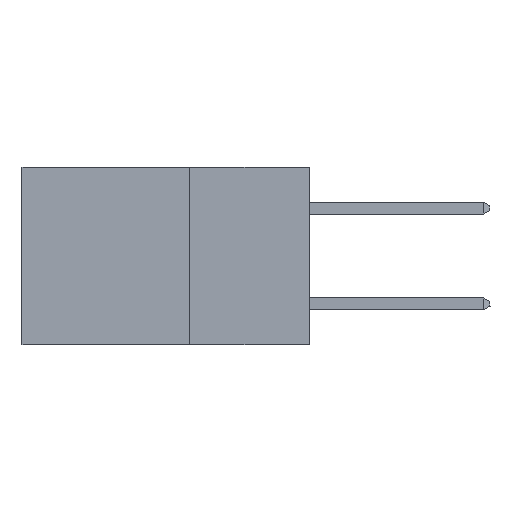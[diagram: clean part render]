
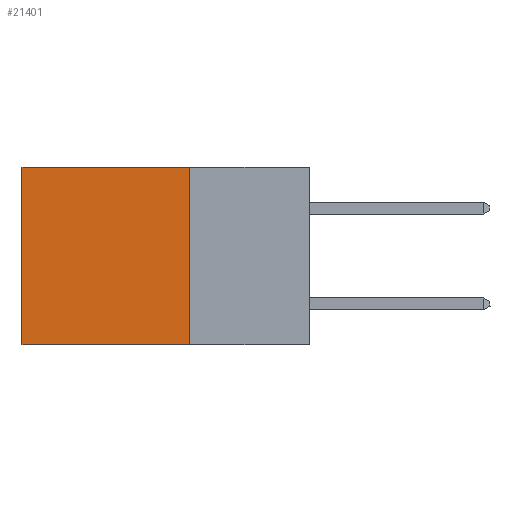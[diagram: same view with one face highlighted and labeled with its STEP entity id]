
A CAD part, left-side view. The second image highlights one B-rep face of the part: STEP entity #21401.
In plain terms, the highlighted planar face has unit normal (-1, 0, 0).
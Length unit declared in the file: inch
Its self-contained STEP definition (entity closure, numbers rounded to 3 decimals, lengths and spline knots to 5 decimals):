
#198 = CARTESIAN_POINT ( 'NONE',  ( 0.2875, 0.25, 0. ) ) ;
#1030 = ORIENTED_EDGE ( 'NONE', *, *, #19675, .T. ) ;
#3338 = ORIENTED_EDGE ( 'NONE', *, *, #15295, .F. ) ;
#3913 = CARTESIAN_POINT ( 'NONE',  ( 0.2875, 0.6, -0.37 ) ) ;
#9298 = EDGE_LOOP ( 'NONE', ( #1030, #3338, #30648, #13749 ) ) ;
#10346 = EDGE_CURVE ( 'NONE', #20838, #15249, #14740, .T. ) ;
#10786 = CARTESIAN_POINT ( 'NONE',  ( 0.2875, 0.6, 0. ) ) ;
#10911 = DIRECTION ( 'NONE',  ( 1., 0., 0. ) ) ;
#11903 = VECTOR ( 'NONE', #14813, 39.37008 ) ;
#13749 = ORIENTED_EDGE ( 'NONE', *, *, #10346, .T. ) ;
#14125 = CARTESIAN_POINT ( 'NONE',  ( 0.2875, 0.25, -0.37 ) ) ;
#14226 = VERTEX_POINT ( 'NONE', #3913 ) ;
#14740 = LINE ( 'NONE', #25241, #15002 ) ;
#14813 = DIRECTION ( 'NONE',  ( 0., 0., -1. ) ) ;
#15002 = VECTOR ( 'NONE', #30594, 39.37008 ) ;
#15249 = VERTEX_POINT ( 'NONE', #33793 ) ;
#15295 = EDGE_CURVE ( 'NONE', #20976, #14226, #29809, .T. ) ;
#15940 = VECTOR ( 'NONE', #29234, 39.37008 ) ;
#16302 = CARTESIAN_POINT ( 'NONE',  ( 0.2875, 0.25, -0.37 ) ) ;
#16766 = EDGE_CURVE ( 'NONE', #20838, #20976, #22901, .T. ) ;
#19274 = DIRECTION ( 'NONE',  ( 0., 1., 0. ) ) ;
#19576 = AXIS2_PLACEMENT_3D ( 'NONE', #198, #10911, #26599 ) ;
#19675 = EDGE_CURVE ( 'NONE', #15249, #14226, #21966, .T. ) ;
#20838 = VERTEX_POINT ( 'NONE', #30840 ) ;
#20976 = VERTEX_POINT ( 'NONE', #16302 ) ;
#21401 = ADVANCED_FACE ( 'NONE', ( #28683 ), #26277, .F. ) ;
#21966 = LINE ( 'NONE', #10786, #15940 ) ;
#22901 = LINE ( 'NONE', #33071, #11903 ) ;
#25241 = CARTESIAN_POINT ( 'NONE',  ( 0.2875, 0.25, 0. ) ) ;
#25599 = VECTOR ( 'NONE', #19274, 39.37008 ) ;
#26277 = PLANE ( 'NONE',  #19576 ) ;
#26599 = DIRECTION ( 'NONE',  ( 0., 0., -1. ) ) ;
#28683 = FACE_OUTER_BOUND ( 'NONE', #9298, .T. ) ;
#29234 = DIRECTION ( 'NONE',  ( 0., 0., -1. ) ) ;
#29809 = LINE ( 'NONE', #14125, #25599 ) ;
#30594 = DIRECTION ( 'NONE',  ( 0., 1., 0. ) ) ;
#30648 = ORIENTED_EDGE ( 'NONE', *, *, #16766, .F. ) ;
#30840 = CARTESIAN_POINT ( 'NONE',  ( 0.2875, 0.25, 0. ) ) ;
#33071 = CARTESIAN_POINT ( 'NONE',  ( 0.2875, 0.25, 0. ) ) ;
#33793 = CARTESIAN_POINT ( 'NONE',  ( 0.2875, 0.6, 0. ) ) ;
